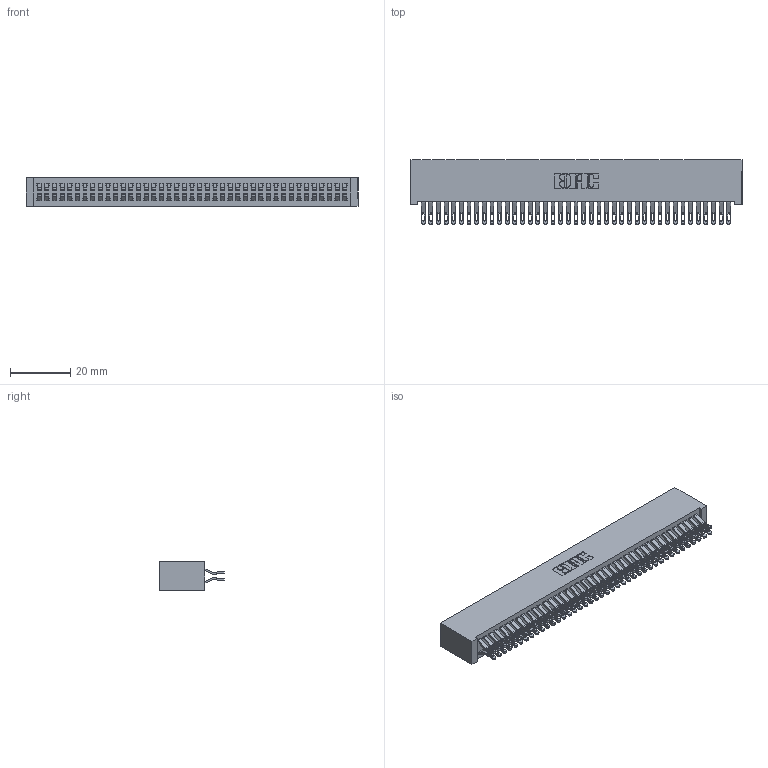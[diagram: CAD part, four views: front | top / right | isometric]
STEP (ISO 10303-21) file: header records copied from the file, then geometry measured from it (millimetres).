
FILE_DESCRIPTION (( 'STEP AP203' ), '1' );
FILE_NAME ('392-082-555-201.STEP', '2018-08-18T03:52:28', ( '' ), ( '' ), 'SwSTEP 2.0', 'SolidWorks 2016', '' );
FILE_SCHEMA (( 'CONFIG_CONTROL_DESIGN' ));
Length unit declared in the file: inch
Products named in the file (3): 392-082-555-201; 342 Part_Lugless; 345-292-001_555 Tail
Assembly tree (83 placements, depth 2):
  392-082-555-201
    342 Part_Lugless
    345-292-001_555 Tail  x82
Bounding box: 110.39 x 21.47 x 9.4 mm (x, y, z)
Volume: 10581 mm3; surface area: 18438.3 mm2
Topology: 83 solids, 83 shells, 4858 faces, 15281 edges, 10186 vertices
Faces by surface type: plane 2850, cylinder 2008
Entity records: 26423 total; most frequent: CARTESIAN_POINT 4412, ORIENTED_EDGE 4318, DIRECTION 3735, EDGE_CURVE 2159, VECTOR 2019, LINE 2019, VERTEX_POINT 1438, AXIS2_PLACEMENT_3D 858
